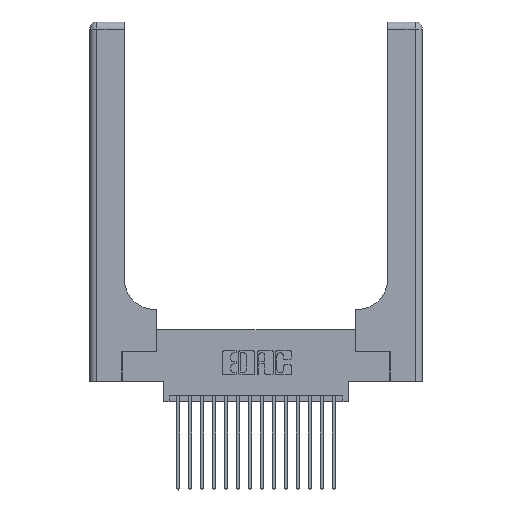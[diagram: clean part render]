
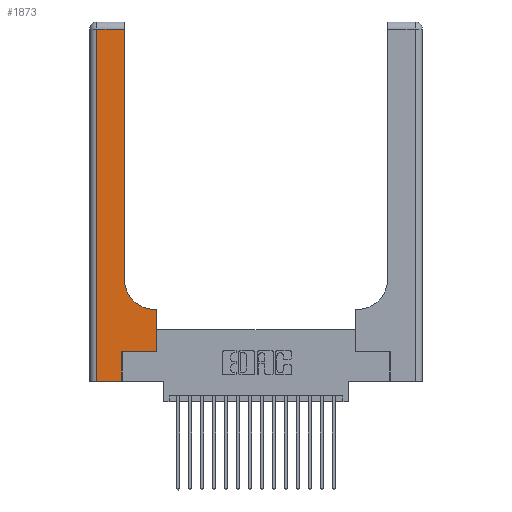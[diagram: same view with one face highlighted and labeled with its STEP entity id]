
A CAD part, top view. The second image highlights one B-rep face of the part: STEP entity #1873.
In plain terms, the highlighted planar face has unit normal (0, 0, 1).
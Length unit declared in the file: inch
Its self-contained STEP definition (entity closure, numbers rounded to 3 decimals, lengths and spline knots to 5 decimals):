
#86 = CARTESIAN_POINT ( 'NONE',  ( 0.2915, 0.6, 0.37 ) ) ;
#219 = ORIENTED_EDGE ( 'NONE', *, *, #5718, .T. ) ;
#336 = ORIENTED_EDGE ( 'NONE', *, *, #5756, .T. ) ;
#625 = VERTEX_POINT ( 'NONE', #675 ) ;
#675 = CARTESIAN_POINT ( 'NONE',  ( 0.2915, 0.85, 0.37 ) ) ;
#1444 = VECTOR ( 'NONE', #18878, 39.37008 ) ;
#1873 = ADVANCED_FACE ( 'NONE', ( #10397 ), #19700, .F. ) ;
#1909 = VECTOR ( 'NONE', #14815, 39.37008 ) ;
#1979 = VECTOR ( 'NONE', #17943, 39.37008 ) ;
#2719 = CARTESIAN_POINT ( 'NONE',  ( 0.5415, 0.6, 0.37 ) ) ;
#3249 = VERTEX_POINT ( 'NONE', #8637 ) ;
#3281 = EDGE_CURVE ( 'NONE', #12109, #8871, #19906, .T. ) ;
#3300 = CARTESIAN_POINT ( 'NONE',  ( 0.06, 0., 0.37 ) ) ;
#3371 = LINE ( 'NONE', #8583, #1909 ) ;
#3393 = CARTESIAN_POINT ( 'NONE',  ( 0.5585, 0.25, 0.37 ) ) ;
#3644 = VECTOR ( 'NONE', #18572, 39.37008 ) ;
#3859 = CARTESIAN_POINT ( 'NONE',  ( 0.5415, 0.85, 0.37 ) ) ;
#4146 = DIRECTION ( 'NONE',  ( -1., 0., 0. ) ) ;
#4934 = CARTESIAN_POINT ( 'NONE',  ( 0.269, 0.25, 0.37 ) ) ;
#5050 = DIRECTION ( 'NONE',  ( 0., 1., 0. ) ) ;
#5084 = ORIENTED_EDGE ( 'NONE', *, *, #3281, .T. ) ;
#5088 = EDGE_CURVE ( 'NONE', #3249, #8310, #20108, .T. ) ;
#5361 = ORIENTED_EDGE ( 'NONE', *, *, #18036, .T. ) ;
#5391 = VECTOR ( 'NONE', #13444, 39.37008 ) ;
#5718 = EDGE_CURVE ( 'NONE', #13775, #3249, #15734, .T. ) ;
#5756 = EDGE_CURVE ( 'NONE', #625, #12109, #9709, .T. ) ;
#6142 = EDGE_CURVE ( 'NONE', #8310, #625, #7011, .T. ) ;
#6247 = DIRECTION ( 'NONE',  ( 1., 0., 0. ) ) ;
#6451 = AXIS2_PLACEMENT_3D ( 'NONE', #3859, #14974, #16232 ) ;
#6589 = CARTESIAN_POINT ( 'NONE',  ( 0.2915, 3., 0.37 ) ) ;
#7011 = CIRCLE ( 'NONE', #6451, 0.25 ) ;
#8310 = VERTEX_POINT ( 'NONE', #2719 ) ;
#8583 = CARTESIAN_POINT ( 'NONE',  ( 0.06, 3., 0.37 ) ) ;
#8637 = CARTESIAN_POINT ( 'NONE',  ( 0.5585, 0.6, 0.37 ) ) ;
#8716 = EDGE_CURVE ( 'NONE', #11976, #18176, #19223, .T. ) ;
#8834 = ORIENTED_EDGE ( 'NONE', *, *, #6142, .T. ) ;
#8871 = VERTEX_POINT ( 'NONE', #19060 ) ;
#8973 = EDGE_LOOP ( 'NONE', ( #336, #5084, #5361, #15402, #11478, #16111, #219, #13308, #8834 ) ) ;
#9517 = CARTESIAN_POINT ( 'NONE',  ( 0., 0., 0.37 ) ) ;
#9709 = LINE ( 'NONE', #6589, #1444 ) ;
#10262 = CARTESIAN_POINT ( 'NONE',  ( 0., 2.94, 0.37 ) ) ;
#10396 = LINE ( 'NONE', #18508, #16418 ) ;
#10397 = FACE_OUTER_BOUND ( 'NONE', #8973, .T. ) ;
#11446 = LINE ( 'NONE', #16405, #1979 ) ;
#11478 = ORIENTED_EDGE ( 'NONE', *, *, #13051, .T. ) ;
#11499 = AXIS2_PLACEMENT_3D ( 'NONE', #13458, #17997, #4146 ) ;
#11663 = VECTOR ( 'NONE', #5050, 39.37008 ) ;
#11976 = VERTEX_POINT ( 'NONE', #3300 ) ;
#12109 = VERTEX_POINT ( 'NONE', #19315 ) ;
#12954 = CARTESIAN_POINT ( 'NONE',  ( 0.5585, 0.25, 0.37 ) ) ;
#13051 = EDGE_CURVE ( 'NONE', #18176, #16041, #10396, .T. ) ;
#13308 = ORIENTED_EDGE ( 'NONE', *, *, #5088, .T. ) ;
#13444 = DIRECTION ( 'NONE',  ( -1., 0., 0. ) ) ;
#13458 = CARTESIAN_POINT ( 'NONE',  ( 0., 3., 0.37 ) ) ;
#13775 = VERTEX_POINT ( 'NONE', #3393 ) ;
#14008 = DIRECTION ( 'NONE',  ( 0., 1., 0. ) ) ;
#14815 = DIRECTION ( 'NONE',  ( 0., -1., 0. ) ) ;
#14974 = DIRECTION ( 'NONE',  ( 0., 0., -1. ) ) ;
#15330 = CARTESIAN_POINT ( 'NONE',  ( 0.269, 0., 0.37 ) ) ;
#15402 = ORIENTED_EDGE ( 'NONE', *, *, #8716, .T. ) ;
#15734 = LINE ( 'NONE', #12954, #11663 ) ;
#15825 = VECTOR ( 'NONE', #6247, 39.37008 ) ;
#16041 = VERTEX_POINT ( 'NONE', #4934 ) ;
#16111 = ORIENTED_EDGE ( 'NONE', *, *, #16333, .T. ) ;
#16232 = DIRECTION ( 'NONE',  ( 1., 0., 0. ) ) ;
#16333 = EDGE_CURVE ( 'NONE', #16041, #13775, #11446, .T. ) ;
#16405 = CARTESIAN_POINT ( 'NONE',  ( 0.269, 0.25, 0.37 ) ) ;
#16418 = VECTOR ( 'NONE', #14008, 39.37008 ) ;
#17943 = DIRECTION ( 'NONE',  ( 1., 0., 0. ) ) ;
#17997 = DIRECTION ( 'NONE',  ( 0., 0., -1. ) ) ;
#18036 = EDGE_CURVE ( 'NONE', #8871, #11976, #3371, .T. ) ;
#18176 = VERTEX_POINT ( 'NONE', #15330 ) ;
#18508 = CARTESIAN_POINT ( 'NONE',  ( 0.269, 0., 0.37 ) ) ;
#18572 = DIRECTION ( 'NONE',  ( -1., 0., 0. ) ) ;
#18878 = DIRECTION ( 'NONE',  ( 0., 1., 0. ) ) ;
#19060 = CARTESIAN_POINT ( 'NONE',  ( 0.06, 2.94, 0.37 ) ) ;
#19223 = LINE ( 'NONE', #9517, #15825 ) ;
#19315 = CARTESIAN_POINT ( 'NONE',  ( 0.2915, 2.94, 0.37 ) ) ;
#19700 = PLANE ( 'NONE',  #11499 ) ;
#19906 = LINE ( 'NONE', #10262, #5391 ) ;
#20108 = LINE ( 'NONE', #86, #3644 ) ;
